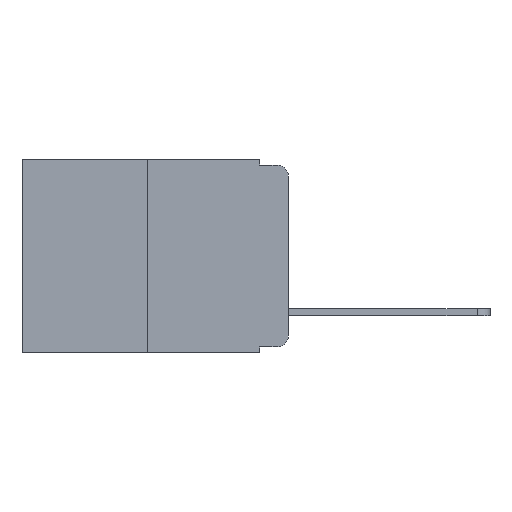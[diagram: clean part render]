
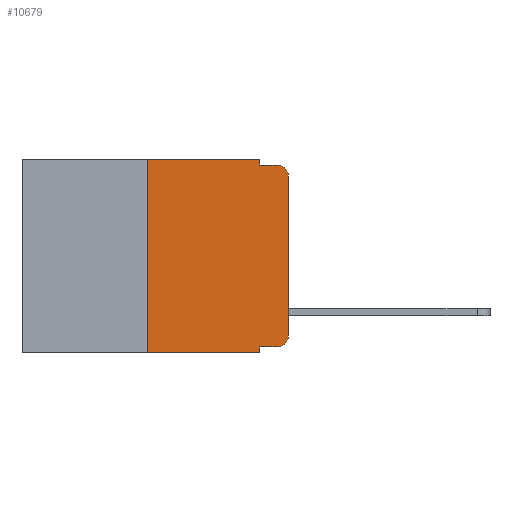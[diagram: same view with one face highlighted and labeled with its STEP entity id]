
A CAD part, left-side view. The second image highlights one B-rep face of the part: STEP entity #10679.
In plain terms, the highlighted planar face has unit normal (-1, 0, 0).
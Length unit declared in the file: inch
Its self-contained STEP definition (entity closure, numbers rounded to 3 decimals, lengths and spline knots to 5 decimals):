
#689 = VERTEX_POINT ( 'NONE', #8498 ) ;
#727 = CARTESIAN_POINT ( 'NONE',  ( 0., 0.25, -0.343 ) ) ;
#1442 = LINE ( 'NONE', #7390, #3971 ) ;
#1496 = CARTESIAN_POINT ( 'NONE',  ( 0., 0., -0.313 ) ) ;
#1828 = ORIENTED_EDGE ( 'NONE', *, *, #9330, .F. ) ;
#1955 = VERTEX_POINT ( 'NONE', #3227 ) ;
#2209 = ORIENTED_EDGE ( 'NONE', *, *, #4249, .F. ) ;
#2228 = LINE ( 'NONE', #12443, #13368 ) ;
#2546 = DIRECTION ( 'NONE',  ( 0., 0., -1. ) ) ;
#2599 = ORIENTED_EDGE ( 'NONE', *, *, #4153, .T. ) ;
#3052 = EDGE_LOOP ( 'NONE', ( #9391, #12146, #6728, #9714, #13356, #1828, #8150, #2209, #11357, #2599 ) ) ;
#3082 = AXIS2_PLACEMENT_3D ( 'NONE', #8754, #11924, #5324 ) ;
#3227 = CARTESIAN_POINT ( 'NONE',  ( 0., 0.051, -0.01 ) ) ;
#3307 = FACE_OUTER_BOUND ( 'NONE', #3052, .T. ) ;
#3517 = CARTESIAN_POINT ( 'NONE',  ( 0., 0.02, -0.313 ) ) ;
#3971 = VECTOR ( 'NONE', #7347, 39.37008 ) ;
#4032 = EDGE_CURVE ( 'NONE', #1955, #13185, #5966, .T. ) ;
#4091 = CARTESIAN_POINT ( 'NONE',  ( 0., 0.25, 0. ) ) ;
#4093 = VERTEX_POINT ( 'NONE', #13293 ) ;
#4115 = PLANE ( 'NONE',  #3082 ) ;
#4153 = EDGE_CURVE ( 'NONE', #689, #11339, #9196, .T. ) ;
#4249 = EDGE_CURVE ( 'NONE', #4093, #4659, #13385, .T. ) ;
#4268 = EDGE_CURVE ( 'NONE', #4740, #1955, #8184, .T. ) ;
#4298 = EDGE_CURVE ( 'NONE', #11339, #13129, #1442, .T. ) ;
#4315 = EDGE_CURVE ( 'NONE', #13129, #13185, #10067, .T. ) ;
#4442 = EDGE_CURVE ( 'NONE', #14099, #4740, #13229, .T. ) ;
#4547 = VECTOR ( 'NONE', #5367, 39.37008 ) ;
#4577 = EDGE_CURVE ( 'NONE', #4093, #689, #2228, .T. ) ;
#4659 = VERTEX_POINT ( 'NONE', #8421 ) ;
#4740 = VERTEX_POINT ( 'NONE', #9726 ) ;
#4757 = DIRECTION ( 'NONE',  ( 0., 0., -1. ) ) ;
#5305 = DIRECTION ( 'NONE',  ( 0., 0., 1. ) ) ;
#5324 = DIRECTION ( 'NONE',  ( 0., 0., -1. ) ) ;
#5326 = LINE ( 'NONE', #4091, #14119 ) ;
#5367 = DIRECTION ( 'NONE',  ( 0., -1., 0. ) ) ;
#5372 = VECTOR ( 'NONE', #10847, 39.37008 ) ;
#5506 = CARTESIAN_POINT ( 'NONE',  ( 0., 0., -0.03 ) ) ;
#5966 = LINE ( 'NONE', #14094, #11170 ) ;
#6287 = DIRECTION ( 'NONE',  ( -1., 0., 0. ) ) ;
#6728 = ORIENTED_EDGE ( 'NONE', *, *, #4032, .F. ) ;
#7250 = EDGE_CURVE ( 'NONE', #11670, #4659, #12548, .T. ) ;
#7347 = DIRECTION ( 'NONE',  ( 0., 0., 1. ) ) ;
#7390 = CARTESIAN_POINT ( 'NONE',  ( 0., 0., 0. ) ) ;
#8150 = ORIENTED_EDGE ( 'NONE', *, *, #7250, .T. ) ;
#8184 = LINE ( 'NONE', #8433, #13083 ) ;
#8421 = CARTESIAN_POINT ( 'NONE',  ( 0., 0.051, -0.343 ) ) ;
#8433 = CARTESIAN_POINT ( 'NONE',  ( 0., 0.051, 0. ) ) ;
#8498 = CARTESIAN_POINT ( 'NONE',  ( 0., 0.02, -0.333 ) ) ;
#8653 = CARTESIAN_POINT ( 'NONE',  ( 0., 0.25, 0. ) ) ;
#8754 = CARTESIAN_POINT ( 'NONE',  ( 0., 0.473, 0. ) ) ;
#9196 = CIRCLE ( 'NONE', #13048, 0.02 ) ;
#9330 = EDGE_CURVE ( 'NONE', #11670, #14099, #5326, .T. ) ;
#9391 = ORIENTED_EDGE ( 'NONE', *, *, #4298, .T. ) ;
#9520 = DIRECTION ( 'NONE',  ( 0., 0., -1. ) ) ;
#9714 = ORIENTED_EDGE ( 'NONE', *, *, #4268, .F. ) ;
#9726 = CARTESIAN_POINT ( 'NONE',  ( 0., 0.051, 0. ) ) ;
#9963 = CARTESIAN_POINT ( 'NONE',  ( 0., 0.473, 0. ) ) ;
#10067 = CIRCLE ( 'NONE', #10070, 0.02 ) ;
#10070 = AXIS2_PLACEMENT_3D ( 'NONE', #12737, #6287, #13700 ) ;
#10679 = ADVANCED_FACE ( 'NONE', ( #3307 ), #4115, .F. ) ;
#10742 = VECTOR ( 'NONE', #9520, 39.37008 ) ;
#10847 = DIRECTION ( 'NONE',  ( 0., -1., 0. ) ) ;
#11170 = VECTOR ( 'NONE', #12198, 39.37008 ) ;
#11339 = VERTEX_POINT ( 'NONE', #1496 ) ;
#11357 = ORIENTED_EDGE ( 'NONE', *, *, #4577, .T. ) ;
#11443 = DIRECTION ( 'NONE',  ( -1., 0., 0. ) ) ;
#11572 = CARTESIAN_POINT ( 'NONE',  ( 0., 0.051, 0. ) ) ;
#11670 = VERTEX_POINT ( 'NONE', #727 ) ;
#11924 = DIRECTION ( 'NONE',  ( 1., 0., 0. ) ) ;
#12146 = ORIENTED_EDGE ( 'NONE', *, *, #4315, .T. ) ;
#12198 = DIRECTION ( 'NONE',  ( 0., -1., 0. ) ) ;
#12443 = CARTESIAN_POINT ( 'NONE',  ( 0., 0.051, -0.333 ) ) ;
#12548 = LINE ( 'NONE', #12842, #5372 ) ;
#12737 = CARTESIAN_POINT ( 'NONE',  ( 0., 0.02, -0.03 ) ) ;
#12842 = CARTESIAN_POINT ( 'NONE',  ( 0., 0.473, -0.343 ) ) ;
#13009 = CARTESIAN_POINT ( 'NONE',  ( 0., 0.02, -0.01 ) ) ;
#13048 = AXIS2_PLACEMENT_3D ( 'NONE', #3517, #11443, #4757 ) ;
#13083 = VECTOR ( 'NONE', #2546, 39.37008 ) ;
#13129 = VERTEX_POINT ( 'NONE', #5506 ) ;
#13185 = VERTEX_POINT ( 'NONE', #13009 ) ;
#13229 = LINE ( 'NONE', #9963, #4547 ) ;
#13293 = CARTESIAN_POINT ( 'NONE',  ( 0., 0.051, -0.333 ) ) ;
#13356 = ORIENTED_EDGE ( 'NONE', *, *, #4442, .F. ) ;
#13368 = VECTOR ( 'NONE', #14287, 39.37008 ) ;
#13385 = LINE ( 'NONE', #11572, #10742 ) ;
#13700 = DIRECTION ( 'NONE',  ( 0., 0., -1. ) ) ;
#14094 = CARTESIAN_POINT ( 'NONE',  ( 0., 0.051, -0.01 ) ) ;
#14099 = VERTEX_POINT ( 'NONE', #8653 ) ;
#14119 = VECTOR ( 'NONE', #5305, 39.37008 ) ;
#14287 = DIRECTION ( 'NONE',  ( 0., -1., 0. ) ) ;
